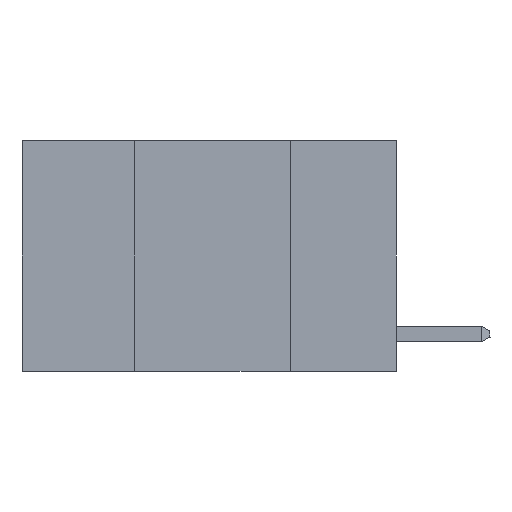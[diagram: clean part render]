
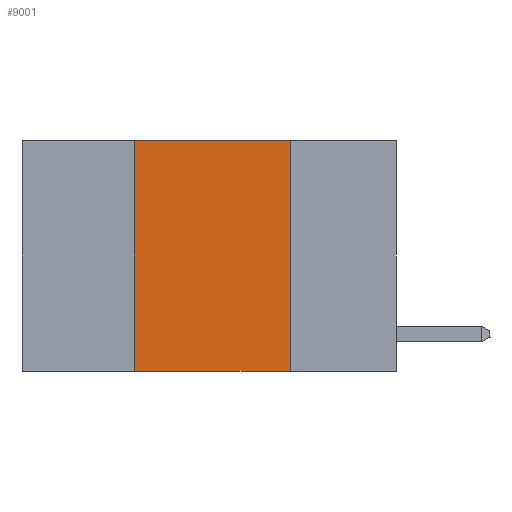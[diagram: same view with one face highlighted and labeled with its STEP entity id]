
A CAD part, left-side view. The second image highlights one B-rep face of the part: STEP entity #9001.
In plain terms, the highlighted planar face has unit normal (-1, 0, 0).
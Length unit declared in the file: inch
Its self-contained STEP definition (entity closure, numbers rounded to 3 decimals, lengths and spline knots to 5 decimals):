
#18 = VERTEX_POINT ( 'NONE', #14295 ) ;
#956 = VECTOR ( 'NONE', #3618, 39.37008 ) ;
#1121 = LINE ( 'NONE', #16398, #16694 ) ;
#1841 = CARTESIAN_POINT ( 'NONE',  ( 0., 0.6, 0. ) ) ;
#3048 = DIRECTION ( 'NONE',  ( 0., 0., 1. ) ) ;
#3399 = PLANE ( 'NONE',  #16838 ) ;
#3618 = DIRECTION ( 'NONE',  ( 0., 0., -1. ) ) ;
#3947 = EDGE_LOOP ( 'NONE', ( #17278, #6315, #14367, #11815 ) ) ;
#4265 = LINE ( 'NONE', #16814, #7874 ) ;
#4359 = LINE ( 'NONE', #10684, #8903 ) ;
#4948 = DIRECTION ( 'NONE',  ( 1., 0., 0. ) ) ;
#5669 = VERTEX_POINT ( 'NONE', #14360 ) ;
#6315 = ORIENTED_EDGE ( 'NONE', *, *, #18166, .F. ) ;
#7629 = CARTESIAN_POINT ( 'NONE',  ( 0., 0.17, -0.37 ) ) ;
#7874 = VECTOR ( 'NONE', #10873, 39.37008 ) ;
#8195 = EDGE_CURVE ( 'NONE', #5669, #18, #4359, .T. ) ;
#8903 = VECTOR ( 'NONE', #3048, 39.37008 ) ;
#8962 = DIRECTION ( 'NONE',  ( 0., -1., 0. ) ) ;
#9001 = ADVANCED_FACE ( 'NONE', ( #13874 ), #3399, .F. ) ;
#9078 = LINE ( 'NONE', #17211, #956 ) ;
#9896 = VERTEX_POINT ( 'NONE', #10461 ) ;
#10248 = EDGE_CURVE ( 'NONE', #9896, #17685, #9078, .T. ) ;
#10461 = CARTESIAN_POINT ( 'NONE',  ( 0., 0.17, 0. ) ) ;
#10684 = CARTESIAN_POINT ( 'NONE',  ( 0., 0.42, 0. ) ) ;
#10873 = DIRECTION ( 'NONE',  ( 0., -1., 0. ) ) ;
#11815 = ORIENTED_EDGE ( 'NONE', *, *, #12774, .T. ) ;
#12774 = EDGE_CURVE ( 'NONE', #5669, #17685, #1121, .T. ) ;
#13874 = FACE_OUTER_BOUND ( 'NONE', #3947, .T. ) ;
#14295 = CARTESIAN_POINT ( 'NONE',  ( 0., 0.42, 0. ) ) ;
#14360 = CARTESIAN_POINT ( 'NONE',  ( 0., 0.42, -0.37 ) ) ;
#14367 = ORIENTED_EDGE ( 'NONE', *, *, #8195, .F. ) ;
#15508 = DIRECTION ( 'NONE',  ( 0., 0., -1. ) ) ;
#16398 = CARTESIAN_POINT ( 'NONE',  ( 0., 0.6, -0.37 ) ) ;
#16694 = VECTOR ( 'NONE', #8962, 39.37008 ) ;
#16814 = CARTESIAN_POINT ( 'NONE',  ( 0., 0.6, 0. ) ) ;
#16838 = AXIS2_PLACEMENT_3D ( 'NONE', #1841, #4948, #15508 ) ;
#17211 = CARTESIAN_POINT ( 'NONE',  ( 0., 0.17, 0. ) ) ;
#17278 = ORIENTED_EDGE ( 'NONE', *, *, #10248, .F. ) ;
#17685 = VERTEX_POINT ( 'NONE', #7629 ) ;
#18166 = EDGE_CURVE ( 'NONE', #18, #9896, #4265, .T. ) ;
